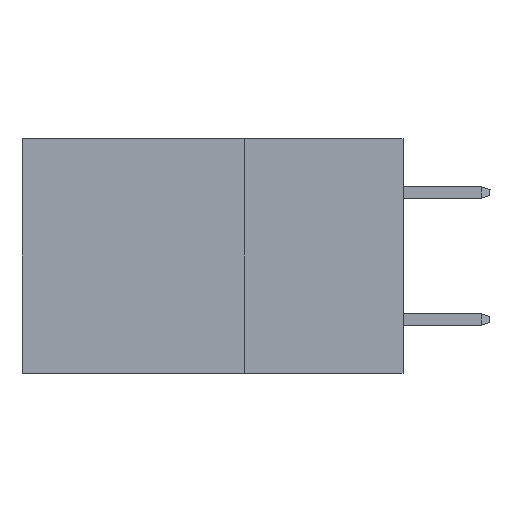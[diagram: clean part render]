
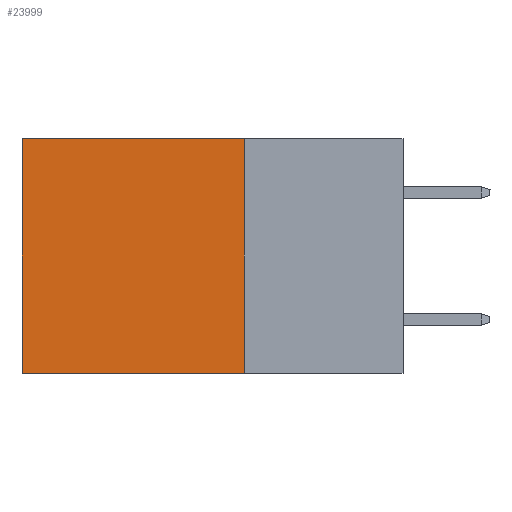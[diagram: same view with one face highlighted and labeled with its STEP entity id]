
A CAD part, left-side view. The second image highlights one B-rep face of the part: STEP entity #23999.
In plain terms, the highlighted planar face has unit normal (-1, 0, 0).
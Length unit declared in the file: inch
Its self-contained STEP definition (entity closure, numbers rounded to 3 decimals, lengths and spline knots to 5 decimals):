
#5275 = CARTESIAN_POINT ( 'NONE',  ( 0.2875, 0.25, -0.37 ) ) ;
#6604 = AXIS2_PLACEMENT_3D ( 'NONE', #24649, #8882, #34257 ) ;
#6774 = VERTEX_POINT ( 'NONE', #15627 ) ;
#8882 = DIRECTION ( 'NONE',  ( 1., 0., 0. ) ) ;
#9791 = LINE ( 'NONE', #21983, #38580 ) ;
#10492 = EDGE_CURVE ( 'NONE', #23293, #28798, #38126, .T. ) ;
#10592 = PLANE ( 'NONE',  #6604 ) ;
#12800 = CARTESIAN_POINT ( 'NONE',  ( 0.2875, 0.25, 0. ) ) ;
#13514 = DIRECTION ( 'NONE',  ( 0., 0., -1. ) ) ;
#15627 = CARTESIAN_POINT ( 'NONE',  ( 0.2875, 0.25, -0.37 ) ) ;
#15675 = CARTESIAN_POINT ( 'NONE',  ( 0.2875, 0.6, -0.37 ) ) ;
#16478 = CARTESIAN_POINT ( 'NONE',  ( 0.2875, 0.25, 0. ) ) ;
#18852 = EDGE_CURVE ( 'NONE', #6774, #28798, #21235, .T. ) ;
#21235 = LINE ( 'NONE', #5275, #31746 ) ;
#21385 = EDGE_CURVE ( 'NONE', #24712, #6774, #22243, .T. ) ;
#21983 = CARTESIAN_POINT ( 'NONE',  ( 0.2875, 0.25, 0. ) ) ;
#22243 = LINE ( 'NONE', #12800, #29898 ) ;
#23293 = VERTEX_POINT ( 'NONE', #38544 ) ;
#23999 = ADVANCED_FACE ( 'NONE', ( #30498 ), #10592, .F. ) ;
#24649 = CARTESIAN_POINT ( 'NONE',  ( 0.2875, 0.25, 0. ) ) ;
#24712 = VERTEX_POINT ( 'NONE', #16478 ) ;
#27114 = VECTOR ( 'NONE', #13514, 39.37008 ) ;
#28473 = DIRECTION ( 'NONE',  ( 0., 1., 0. ) ) ;
#28798 = VERTEX_POINT ( 'NONE', #15675 ) ;
#29898 = VECTOR ( 'NONE', #31475, 39.37008 ) ;
#30048 = DIRECTION ( 'NONE',  ( 0., 1., 0. ) ) ;
#30498 = FACE_OUTER_BOUND ( 'NONE', #36210, .T. ) ;
#31475 = DIRECTION ( 'NONE',  ( 0., 0., -1. ) ) ;
#31746 = VECTOR ( 'NONE', #30048, 39.37008 ) ;
#31832 = CARTESIAN_POINT ( 'NONE',  ( 0.2875, 0.6, 0. ) ) ;
#33341 = EDGE_CURVE ( 'NONE', #24712, #23293, #9791, .T. ) ;
#34028 = ORIENTED_EDGE ( 'NONE', *, *, #10492, .T. ) ;
#34257 = DIRECTION ( 'NONE',  ( 0., 0., -1. ) ) ;
#34513 = ORIENTED_EDGE ( 'NONE', *, *, #33341, .T. ) ;
#35368 = ORIENTED_EDGE ( 'NONE', *, *, #18852, .F. ) ;
#36210 = EDGE_LOOP ( 'NONE', ( #34028, #35368, #40560, #34513 ) ) ;
#38126 = LINE ( 'NONE', #31832, #27114 ) ;
#38544 = CARTESIAN_POINT ( 'NONE',  ( 0.2875, 0.6, 0. ) ) ;
#38580 = VECTOR ( 'NONE', #28473, 39.37008 ) ;
#40560 = ORIENTED_EDGE ( 'NONE', *, *, #21385, .F. ) ;
